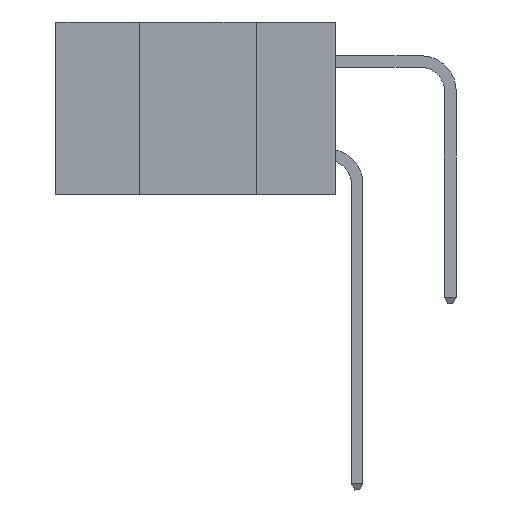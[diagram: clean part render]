
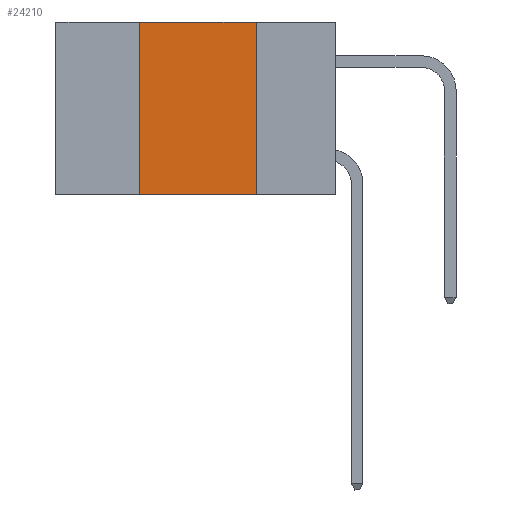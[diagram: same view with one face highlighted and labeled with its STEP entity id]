
A CAD part, left-side view. The second image highlights one B-rep face of the part: STEP entity #24210.
In plain terms, the highlighted planar face has unit normal (-1, 0, 0).
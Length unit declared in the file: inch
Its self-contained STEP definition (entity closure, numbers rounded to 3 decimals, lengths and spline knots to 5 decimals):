
#46 = LINE ( 'NONE', #19938, #5941 ) ;
#2573 = EDGE_CURVE ( 'NONE', #27593, #10121, #30166, .T. ) ;
#3655 = DIRECTION ( 'NONE',  ( 0., 0., 1. ) ) ;
#3882 = CARTESIAN_POINT ( 'NONE',  ( 0., 0.42, -0.37 ) ) ;
#3930 = LINE ( 'NONE', #9237, #9484 ) ;
#4996 = DIRECTION ( 'NONE',  ( 0., -1., 0. ) ) ;
#5598 = ORIENTED_EDGE ( 'NONE', *, *, #21639, .F. ) ;
#5941 = VECTOR ( 'NONE', #4996, 39.37008 ) ;
#6238 = VERTEX_POINT ( 'NONE', #29346 ) ;
#8909 = DIRECTION ( 'NONE',  ( 0., 0., -1. ) ) ;
#9237 = CARTESIAN_POINT ( 'NONE',  ( 0., 0.17, 0. ) ) ;
#9484 = VECTOR ( 'NONE', #8909, 39.37008 ) ;
#9610 = VECTOR ( 'NONE', #3655, 39.37008 ) ;
#10121 = VERTEX_POINT ( 'NONE', #29219 ) ;
#10388 = AXIS2_PLACEMENT_3D ( 'NONE', #24523, #32109, #27267 ) ;
#13294 = CARTESIAN_POINT ( 'NONE',  ( 0., 0.6, 0. ) ) ;
#14013 = ORIENTED_EDGE ( 'NONE', *, *, #25168, .F. ) ;
#16781 = PLANE ( 'NONE',  #10388 ) ;
#19938 = CARTESIAN_POINT ( 'NONE',  ( 0., 0.6, -0.37 ) ) ;
#21043 = EDGE_CURVE ( 'NONE', #27593, #29689, #46, .T. ) ;
#21639 = EDGE_CURVE ( 'NONE', #6238, #29689, #3930, .T. ) ;
#22802 = EDGE_LOOP ( 'NONE', ( #5598, #14013, #29811, #28190 ) ) ;
#24210 = ADVANCED_FACE ( 'NONE', ( #28913 ), #16781, .F. ) ;
#24523 = CARTESIAN_POINT ( 'NONE',  ( 0., 0.6, 0. ) ) ;
#25126 = CARTESIAN_POINT ( 'NONE',  ( 0., 0.17, -0.37 ) ) ;
#25168 = EDGE_CURVE ( 'NONE', #10121, #6238, #32385, .T. ) ;
#25657 = VECTOR ( 'NONE', #28104, 39.37008 ) ;
#27267 = DIRECTION ( 'NONE',  ( 0., 0., -1. ) ) ;
#27593 = VERTEX_POINT ( 'NONE', #3882 ) ;
#28104 = DIRECTION ( 'NONE',  ( 0., -1., 0. ) ) ;
#28190 = ORIENTED_EDGE ( 'NONE', *, *, #21043, .T. ) ;
#28913 = FACE_OUTER_BOUND ( 'NONE', #22802, .T. ) ;
#29219 = CARTESIAN_POINT ( 'NONE',  ( 0., 0.42, 0. ) ) ;
#29346 = CARTESIAN_POINT ( 'NONE',  ( 0., 0.17, 0. ) ) ;
#29689 = VERTEX_POINT ( 'NONE', #25126 ) ;
#29811 = ORIENTED_EDGE ( 'NONE', *, *, #2573, .F. ) ;
#30166 = LINE ( 'NONE', #31033, #9610 ) ;
#31033 = CARTESIAN_POINT ( 'NONE',  ( 0., 0.42, 0. ) ) ;
#32109 = DIRECTION ( 'NONE',  ( 1., 0., 0. ) ) ;
#32385 = LINE ( 'NONE', #13294, #25657 ) ;
